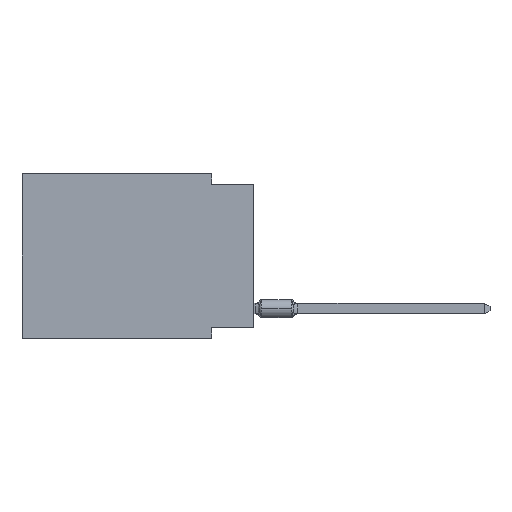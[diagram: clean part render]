
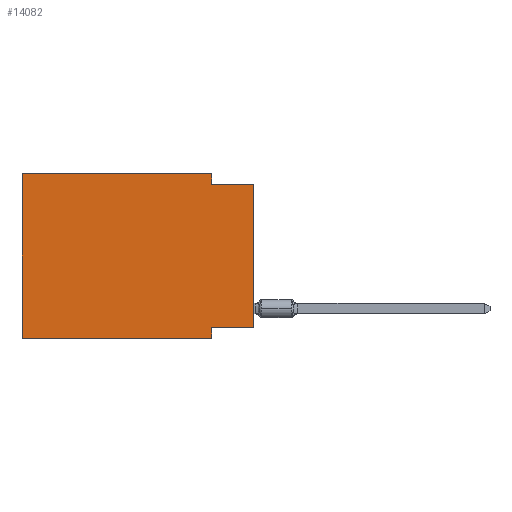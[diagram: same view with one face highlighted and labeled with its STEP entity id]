
A CAD part, left-side view. The second image highlights one B-rep face of the part: STEP entity #14082.
In plain terms, the highlighted planar face has unit normal (-1, 0, 0).
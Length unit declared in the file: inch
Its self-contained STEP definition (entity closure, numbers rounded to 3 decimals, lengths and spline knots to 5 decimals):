
#127 = LINE ( 'NONE', #11524, #15891 ) ;
#471 = ORIENTED_EDGE ( 'NONE', *, *, #17257, .F. ) ;
#543 = DIRECTION ( 'NONE',  ( 0., 0., -1. ) ) ;
#750 = VECTOR ( 'NONE', #6592, 39.37008 ) ;
#817 = EDGE_CURVE ( 'NONE', #2613, #8979, #5114, .T. ) ;
#1089 = ORIENTED_EDGE ( 'NONE', *, *, #10958, .F. ) ;
#2407 = ORIENTED_EDGE ( 'NONE', *, *, #817, .F. ) ;
#2613 = VERTEX_POINT ( 'NONE', #13270 ) ;
#2823 = ORIENTED_EDGE ( 'NONE', *, *, #12850, .T. ) ;
#2860 = PLANE ( 'NONE',  #15005 ) ;
#3180 = EDGE_LOOP ( 'NONE', ( #16734, #17488, #1089, #12036, #2407, #2823, #5828, #471 ) ) ;
#3493 = EDGE_CURVE ( 'NONE', #6303, #6027, #14705, .T. ) ;
#4251 = VERTEX_POINT ( 'NONE', #14292 ) ;
#4990 = LINE ( 'NONE', #17742, #14635 ) ;
#5114 = LINE ( 'NONE', #17684, #750 ) ;
#5240 = EDGE_CURVE ( 'NONE', #5479, #6027, #16160, .T. ) ;
#5479 = VERTEX_POINT ( 'NONE', #10053 ) ;
#5589 = VECTOR ( 'NONE', #16868, 39.37008 ) ;
#5605 = CARTESIAN_POINT ( 'NONE',  ( 0., 0.55, 0. ) ) ;
#5828 = ORIENTED_EDGE ( 'NONE', *, *, #7795, .F. ) ;
#6027 = VERTEX_POINT ( 'NONE', #17413 ) ;
#6075 = VERTEX_POINT ( 'NONE', #9092 ) ;
#6303 = VERTEX_POINT ( 'NONE', #17342 ) ;
#6592 = DIRECTION ( 'NONE',  ( 0., 0., 1. ) ) ;
#7077 = CARTESIAN_POINT ( 'NONE',  ( 0., 0., -0.365 ) ) ;
#7795 = EDGE_CURVE ( 'NONE', #6075, #4251, #127, .T. ) ;
#7811 = CARTESIAN_POINT ( 'NONE',  ( 0., 0.55, -0.39 ) ) ;
#8979 = VERTEX_POINT ( 'NONE', #12626 ) ;
#8994 = EDGE_CURVE ( 'NONE', #8979, #12806, #18261, .T. ) ;
#9041 = DIRECTION ( 'NONE',  ( 0., -1., 0. ) ) ;
#9092 = CARTESIAN_POINT ( 'NONE',  ( 0., 0.1, -0.365 ) ) ;
#9286 = LINE ( 'NONE', #7811, #13510 ) ;
#10053 = CARTESIAN_POINT ( 'NONE',  ( 0., 0.1, -0.025 ) ) ;
#10958 = EDGE_CURVE ( 'NONE', #12806, #5479, #4990, .T. ) ;
#11429 = DIRECTION ( 'NONE',  ( 0., 0., -1. ) ) ;
#11465 = CARTESIAN_POINT ( 'NONE',  ( 0., 0.55, 0. ) ) ;
#11524 = CARTESIAN_POINT ( 'NONE',  ( 0., 0.1, -0.39 ) ) ;
#11668 = VECTOR ( 'NONE', #9041, 39.37008 ) ;
#12036 = ORIENTED_EDGE ( 'NONE', *, *, #8994, .F. ) ;
#12112 = CARTESIAN_POINT ( 'NONE',  ( 0., 0., 0. ) ) ;
#12626 = CARTESIAN_POINT ( 'NONE',  ( 0., 0.55, 0. ) ) ;
#12806 = VERTEX_POINT ( 'NONE', #16129 ) ;
#12850 = EDGE_CURVE ( 'NONE', #2613, #4251, #9286, .T. ) ;
#12934 = DIRECTION ( 'NONE',  ( 0., 0., -1. ) ) ;
#13270 = CARTESIAN_POINT ( 'NONE',  ( 0., 0.55, -0.39 ) ) ;
#13510 = VECTOR ( 'NONE', #14926, 39.37008 ) ;
#14082 = ADVANCED_FACE ( 'NONE', ( #16867 ), #2860, .F. ) ;
#14292 = CARTESIAN_POINT ( 'NONE',  ( 0., 0.1, -0.39 ) ) ;
#14635 = VECTOR ( 'NONE', #543, 39.37008 ) ;
#14705 = LINE ( 'NONE', #12112, #14821 ) ;
#14797 = DIRECTION ( 'NONE',  ( 0., 0., 1. ) ) ;
#14821 = VECTOR ( 'NONE', #14797, 39.37008 ) ;
#14926 = DIRECTION ( 'NONE',  ( 0., -1., 0. ) ) ;
#15005 = AXIS2_PLACEMENT_3D ( 'NONE', #11465, #15428, #12934 ) ;
#15428 = DIRECTION ( 'NONE',  ( 1., 0., 0. ) ) ;
#15485 = DIRECTION ( 'NONE',  ( 0., -1., 0. ) ) ;
#15548 = VECTOR ( 'NONE', #15485, 39.37008 ) ;
#15891 = VECTOR ( 'NONE', #11429, 39.37008 ) ;
#16064 = CARTESIAN_POINT ( 'NONE',  ( 0., 0., -0.025 ) ) ;
#16129 = CARTESIAN_POINT ( 'NONE',  ( 0., 0.1, 0. ) ) ;
#16160 = LINE ( 'NONE', #16064, #11668 ) ;
#16734 = ORIENTED_EDGE ( 'NONE', *, *, #3493, .T. ) ;
#16867 = FACE_OUTER_BOUND ( 'NONE', #3180, .T. ) ;
#16868 = DIRECTION ( 'NONE',  ( 0., 1., 0. ) ) ;
#17257 = EDGE_CURVE ( 'NONE', #6303, #6075, #17972, .T. ) ;
#17342 = CARTESIAN_POINT ( 'NONE',  ( 0., 0., -0.365 ) ) ;
#17413 = CARTESIAN_POINT ( 'NONE',  ( 0., 0., -0.025 ) ) ;
#17488 = ORIENTED_EDGE ( 'NONE', *, *, #5240, .F. ) ;
#17684 = CARTESIAN_POINT ( 'NONE',  ( 0., 0.55, 0. ) ) ;
#17742 = CARTESIAN_POINT ( 'NONE',  ( 0., 0.1, 0. ) ) ;
#17972 = LINE ( 'NONE', #7077, #5589 ) ;
#18261 = LINE ( 'NONE', #5605, #15548 ) ;
